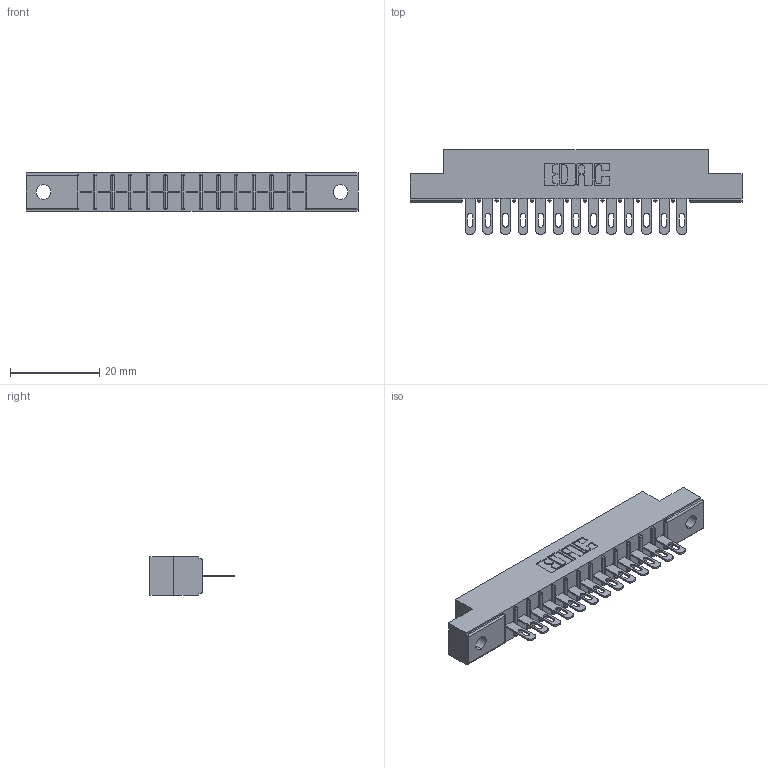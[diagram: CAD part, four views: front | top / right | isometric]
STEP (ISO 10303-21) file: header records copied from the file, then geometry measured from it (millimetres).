
FILE_DESCRIPTION (( 'STEP AP203' ), '1' );
FILE_NAME ('316-013-500-102.STEP', '2018-07-31T00:29:48', ( '' ), ( '' ), 'SwSTEP 2.0', 'SolidWorks 2016', '' );
FILE_SCHEMA (( 'CONFIG_CONTROL_DESIGN' ));
Length unit declared in the file: inch
Products named in the file (3): 316-013-500-102; 306 Part_.128 Dia; 306-290-001_100
Assembly tree (14 placements, depth 2):
  316-013-500-102
    306 Part_.128 Dia
    306-290-001_100  x13
Bounding box: 74.52 x 18.87 x 8.71 mm (x, y, z)
Volume: 5066.2 mm3; surface area: 7143 mm2
Topology: 14 solids, 14 shells, 1104 faces, 3111 edges, 2002 vertices
Faces by surface type: plane 718, cylinder 334, sphere 52
Entity records: 16046 total; most frequent: CARTESIAN_POINT 2690, ORIENTED_EDGE 2662, DIRECTION 2657, EDGE_CURVE 1331, LINE 1023, VECTOR 1023, VERTEX_POINT 850, AXIS2_PLACEMENT_3D 817
